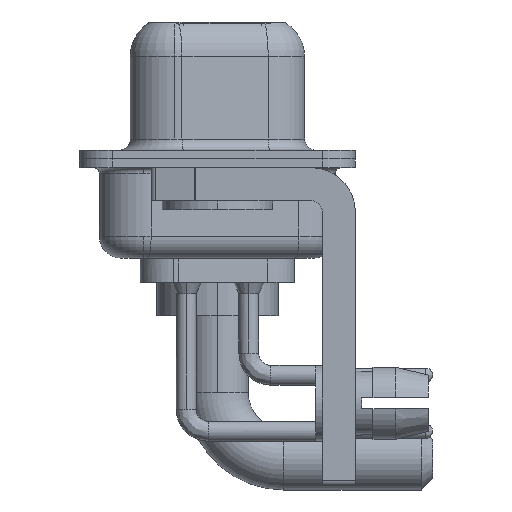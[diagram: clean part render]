
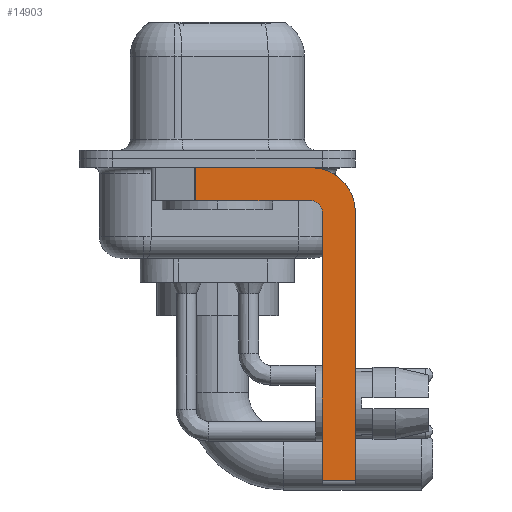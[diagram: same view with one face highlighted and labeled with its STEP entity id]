
A CAD part, left-side view. The second image highlights one B-rep face of the part: STEP entity #14903.
In plain terms, the highlighted planar face has unit normal (-1, 0, 0).
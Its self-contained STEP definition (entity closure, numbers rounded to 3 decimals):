
#481 = CARTESIAN_POINT ( 'NONE',  ( -2.9, -4.25, -1.9 ) ) ;
#576 = CARTESIAN_POINT ( 'NONE',  ( -2.9, -4.25, -14.55 ) ) ;
#1051 = DIRECTION ( 'NONE',  ( 1., 0., 0. ) ) ;
#1293 = CARTESIAN_POINT ( 'NONE',  ( -2.9, -6.25, -2.4 ) ) ;
#1300 = LINE ( 'NONE', #11465, #6561 ) ;
#1301 = DIRECTION ( 'NONE',  ( 0., 0., 1. ) ) ;
#1511 = ORIENTED_EDGE ( 'NONE', *, *, #2650, .F. ) ;
#1754 = CARTESIAN_POINT ( 'NONE',  ( -2.9, -4.75, -2.4 ) ) ;
#1860 = VERTEX_POINT ( 'NONE', #8928 ) ;
#1893 = VERTEX_POINT ( 'NONE', #10455 ) ;
#2275 = VECTOR ( 'NONE', #8530, 1000. ) ;
#2371 = VECTOR ( 'NONE', #17768, 1000. ) ;
#2625 = LINE ( 'NONE', #5735, #8597 ) ;
#2650 = EDGE_CURVE ( 'NONE', #1893, #15723, #2625, .T. ) ;
#3040 = AXIS2_PLACEMENT_3D ( 'NONE', #11115, #1051, #10932 ) ;
#3483 = LINE ( 'NONE', #576, #11152 ) ;
#3598 = EDGE_CURVE ( 'NONE', #1893, #15583, #3483, .T. ) ;
#3630 = DIRECTION ( 'NONE',  ( 1., 0., 0. ) ) ;
#4356 = ORIENTED_EDGE ( 'NONE', *, *, #10289, .F. ) ;
#4561 = ORIENTED_EDGE ( 'NONE', *, *, #7571, .F. ) ;
#4657 = VERTEX_POINT ( 'NONE', #481 ) ;
#4671 = DIRECTION ( 'NONE',  ( 0., 0., 1. ) ) ;
#5287 = CARTESIAN_POINT ( 'NONE',  ( -2.9, 0.978, -1.9 ) ) ;
#5735 = CARTESIAN_POINT ( 'NONE',  ( -2.9, -4.75, -14.8 ) ) ;
#6035 = CIRCLE ( 'NONE', #16644, 0.5 ) ;
#6201 = EDGE_CURVE ( 'NONE', #13433, #15583, #18630, .T. ) ;
#6561 = VECTOR ( 'NONE', #14206, 1000. ) ;
#7199 = EDGE_CURVE ( 'NONE', #1860, #13433, #18625, .T. ) ;
#7571 = EDGE_CURVE ( 'NONE', #13544, #1860, #1300, .T. ) ;
#7636 = CARTESIAN_POINT ( 'NONE',  ( -2.9, -4.25, -2.4 ) ) ;
#8530 = DIRECTION ( 'NONE',  ( 0., 0., -1. ) ) ;
#8597 = VECTOR ( 'NONE', #1301, 1000. ) ;
#8906 = ORIENTED_EDGE ( 'NONE', *, *, #6201, .F. ) ;
#8907 = EDGE_LOOP ( 'NONE', ( #4561, #9402, #4356, #12624, #1511, #15778, #8906, #11435 ) ) ;
#8928 = CARTESIAN_POINT ( 'NONE',  ( -2.9, -4.25, -0.4 ) ) ;
#9293 = DIRECTION ( 'NONE',  ( 0., -1., 0. ) ) ;
#9402 = ORIENTED_EDGE ( 'NONE', *, *, #12877, .T. ) ;
#9878 = FACE_OUTER_BOUND ( 'NONE', #8907, .T. ) ;
#10289 = EDGE_CURVE ( 'NONE', #4657, #13125, #13537, .T. ) ;
#10294 = DIRECTION ( 'NONE',  ( -1., 0., 0. ) ) ;
#10455 = CARTESIAN_POINT ( 'NONE',  ( -2.9, -4.75, -14.55 ) ) ;
#10932 = DIRECTION ( 'NONE',  ( 0., 0., -1. ) ) ;
#11115 = CARTESIAN_POINT ( 'NONE',  ( -2.9, -4.25, -2.4 ) ) ;
#11152 = VECTOR ( 'NONE', #9293, 1000. ) ;
#11435 = ORIENTED_EDGE ( 'NONE', *, *, #7199, .F. ) ;
#11465 = CARTESIAN_POINT ( 'NONE',  ( -2.9, 3., -0.4 ) ) ;
#11478 = CARTESIAN_POINT ( 'NONE',  ( -2.9, -6.25, -2.4 ) ) ;
#11928 = CARTESIAN_POINT ( 'NONE',  ( -2.9, -4.25, -1.9 ) ) ;
#12193 = CARTESIAN_POINT ( 'NONE',  ( -2.9, -4.25, -2.4 ) ) ;
#12520 = LINE ( 'NONE', #5287, #18456 ) ;
#12624 = ORIENTED_EDGE ( 'NONE', *, *, #17545, .F. ) ;
#12877 = EDGE_CURVE ( 'NONE', #13544, #13125, #12520, .T. ) ;
#13125 = VERTEX_POINT ( 'NONE', #13265 ) ;
#13265 = CARTESIAN_POINT ( 'NONE',  ( -2.9, 0.978, -1.9 ) ) ;
#13433 = VERTEX_POINT ( 'NONE', #1293 ) ;
#13537 = LINE ( 'NONE', #11928, #2371 ) ;
#13544 = VERTEX_POINT ( 'NONE', #15807 ) ;
#14206 = DIRECTION ( 'NONE',  ( 0., -1., 0. ) ) ;
#14484 = CARTESIAN_POINT ( 'NONE',  ( -2.9, -6.25, -14.55 ) ) ;
#14727 = AXIS2_PLACEMENT_3D ( 'NONE', #12193, #3630, #17954 ) ;
#14903 = ADVANCED_FACE ( 'NONE', ( #9878 ), #16781, .F. ) ;
#15583 = VERTEX_POINT ( 'NONE', #14484 ) ;
#15723 = VERTEX_POINT ( 'NONE', #1754 ) ;
#15778 = ORIENTED_EDGE ( 'NONE', *, *, #3598, .T. ) ;
#15807 = CARTESIAN_POINT ( 'NONE',  ( -2.9, 0.978, -0.4 ) ) ;
#16644 = AXIS2_PLACEMENT_3D ( 'NONE', #7636, #10294, #4671 ) ;
#16781 = PLANE ( 'NONE',  #3040 ) ;
#16854 = DIRECTION ( 'NONE',  ( 0., 0., -1. ) ) ;
#17545 = EDGE_CURVE ( 'NONE', #15723, #4657, #6035, .T. ) ;
#17768 = DIRECTION ( 'NONE',  ( 0., 1., 0. ) ) ;
#17954 = DIRECTION ( 'NONE',  ( 0., 0., -1. ) ) ;
#18456 = VECTOR ( 'NONE', #16854, 1000. ) ;
#18625 = CIRCLE ( 'NONE', #14727, 2. ) ;
#18630 = LINE ( 'NONE', #11478, #2275 ) ;
